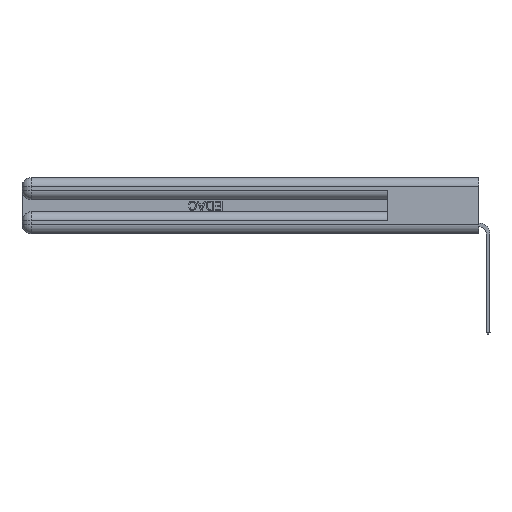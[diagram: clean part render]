
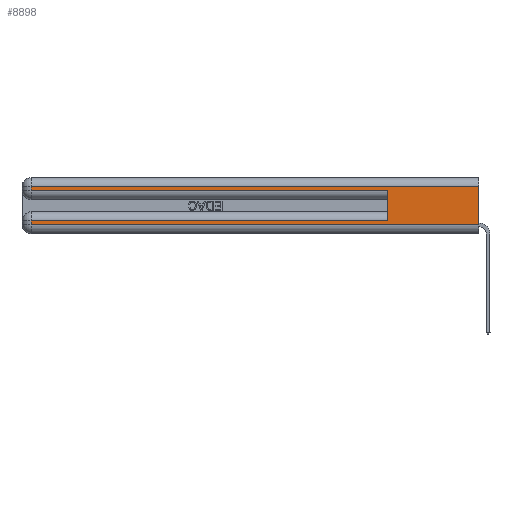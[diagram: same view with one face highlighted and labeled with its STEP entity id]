
A CAD part, left-side view. The second image highlights one B-rep face of the part: STEP entity #8898.
In plain terms, the highlighted planar face has unit normal (-1, 0, 0).
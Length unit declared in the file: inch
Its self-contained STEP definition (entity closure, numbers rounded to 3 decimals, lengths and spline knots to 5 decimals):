
#731 = VECTOR ( 'NONE', #1086, 39.37008 ) ;
#754 = LINE ( 'NONE', #31201, #731 ) ;
#1086 = DIRECTION ( 'NONE',  ( 0., -1., 0. ) ) ;
#1580 = VECTOR ( 'NONE', #26539, 39.37008 ) ;
#1652 = VECTOR ( 'NONE', #16111, 39.37008 ) ;
#2815 = VERTEX_POINT ( 'NONE', #9764 ) ;
#2879 = VERTEX_POINT ( 'NONE', #30800 ) ;
#3183 = CARTESIAN_POINT ( 'NONE',  ( 0., 2.94, 0.37 ) ) ;
#3296 = ORIENTED_EDGE ( 'NONE', *, *, #9941, .F. ) ;
#5044 = VECTOR ( 'NONE', #28785, 39.37008 ) ;
#5956 = CARTESIAN_POINT ( 'NONE',  ( 0., 2.94, 0.31 ) ) ;
#7912 = CARTESIAN_POINT ( 'NONE',  ( 0., 0., 0.31 ) ) ;
#8395 = LINE ( 'NONE', #11097, #14740 ) ;
#8814 = VECTOR ( 'NONE', #30811, 39.37008 ) ;
#8817 = ORIENTED_EDGE ( 'NONE', *, *, #31374, .T. ) ;
#8898 = ADVANCED_FACE ( 'NONE', ( #14857 ), #14365, .F. ) ;
#9433 = EDGE_CURVE ( 'NONE', #32930, #20115, #27789, .T. ) ;
#9615 = EDGE_CURVE ( 'NONE', #2879, #14599, #26417, .T. ) ;
#9764 = CARTESIAN_POINT ( 'NONE',  ( 0., 0.6, 0.085 ) ) ;
#9941 = EDGE_CURVE ( 'NONE', #2815, #30396, #26049, .T. ) ;
#10024 = EDGE_LOOP ( 'NONE', ( #13026, #30872, #8817, #13694, #3296, #11370, #12446, #10367 ) ) ;
#10277 = LINE ( 'NONE', #3183, #19918 ) ;
#10367 = ORIENTED_EDGE ( 'NONE', *, *, #9615, .T. ) ;
#10612 = DIRECTION ( 'NONE',  ( 0., 0., -1. ) ) ;
#11097 = CARTESIAN_POINT ( 'NONE',  ( 0., 0., 0.37 ) ) ;
#11370 = ORIENTED_EDGE ( 'NONE', *, *, #32935, .T. ) ;
#12446 = ORIENTED_EDGE ( 'NONE', *, *, #21096, .T. ) ;
#13026 = ORIENTED_EDGE ( 'NONE', *, *, #23281, .F. ) ;
#13253 = CARTESIAN_POINT ( 'NONE',  ( 0., 0., 0.085 ) ) ;
#13694 = ORIENTED_EDGE ( 'NONE', *, *, #20079, .T. ) ;
#14205 = DIRECTION ( 'NONE',  ( 0., 0., -1. ) ) ;
#14365 = PLANE ( 'NONE',  #15314 ) ;
#14385 = CARTESIAN_POINT ( 'NONE',  ( 0., 0., 0.06 ) ) ;
#14599 = VERTEX_POINT ( 'NONE', #14385 ) ;
#14740 = VECTOR ( 'NONE', #16643, 39.37008 ) ;
#14857 = FACE_OUTER_BOUND ( 'NONE', #10024, .T. ) ;
#15314 = AXIS2_PLACEMENT_3D ( 'NONE', #29678, #24638, #14205 ) ;
#16111 = DIRECTION ( 'NONE',  ( 0., 1., 0. ) ) ;
#16643 = DIRECTION ( 'NONE',  ( 0., 0., -1. ) ) ;
#17469 = CARTESIAN_POINT ( 'NONE',  ( 0., 2.94, 0.37 ) ) ;
#18131 = LINE ( 'NONE', #13253, #1652 ) ;
#19654 = CARTESIAN_POINT ( 'NONE',  ( 0., 2.94, 0.085 ) ) ;
#19894 = VERTEX_POINT ( 'NONE', #28199 ) ;
#19918 = VECTOR ( 'NONE', #10612, 39.37008 ) ;
#20079 = EDGE_CURVE ( 'NONE', #19894, #30396, #754, .T. ) ;
#20115 = VERTEX_POINT ( 'NONE', #5956 ) ;
#20820 = CARTESIAN_POINT ( 'NONE',  ( 0., 0.6, 0.145 ) ) ;
#21096 = EDGE_CURVE ( 'NONE', #23538, #2879, #22354, .T. ) ;
#22354 = LINE ( 'NONE', #17469, #27634 ) ;
#23197 = CARTESIAN_POINT ( 'NONE',  ( 0., 0., 0.31 ) ) ;
#23281 = EDGE_CURVE ( 'NONE', #32930, #14599, #8395, .T. ) ;
#23538 = VERTEX_POINT ( 'NONE', #19654 ) ;
#24638 = DIRECTION ( 'NONE',  ( 1., 0., 0. ) ) ;
#25157 = CARTESIAN_POINT ( 'NONE',  ( 0., 0.6, 0.285 ) ) ;
#26049 = LINE ( 'NONE', #20820, #1580 ) ;
#26417 = LINE ( 'NONE', #31138, #5044 ) ;
#26539 = DIRECTION ( 'NONE',  ( 0., 0., 1. ) ) ;
#27634 = VECTOR ( 'NONE', #32616, 39.37008 ) ;
#27789 = LINE ( 'NONE', #7912, #8814 ) ;
#28199 = CARTESIAN_POINT ( 'NONE',  ( 0., 2.94, 0.285 ) ) ;
#28785 = DIRECTION ( 'NONE',  ( 0., -1., 0. ) ) ;
#29678 = CARTESIAN_POINT ( 'NONE',  ( 0., 0., 0.37 ) ) ;
#30396 = VERTEX_POINT ( 'NONE', #25157 ) ;
#30800 = CARTESIAN_POINT ( 'NONE',  ( 0., 2.94, 0.06 ) ) ;
#30811 = DIRECTION ( 'NONE',  ( 0., 1., 0. ) ) ;
#30872 = ORIENTED_EDGE ( 'NONE', *, *, #9433, .T. ) ;
#31138 = CARTESIAN_POINT ( 'NONE',  ( 0., 0., 0.06 ) ) ;
#31201 = CARTESIAN_POINT ( 'NONE',  ( 0., 0., 0.285 ) ) ;
#31374 = EDGE_CURVE ( 'NONE', #20115, #19894, #10277, .T. ) ;
#32616 = DIRECTION ( 'NONE',  ( 0., 0., -1. ) ) ;
#32930 = VERTEX_POINT ( 'NONE', #23197 ) ;
#32935 = EDGE_CURVE ( 'NONE', #2815, #23538, #18131, .T. ) ;
